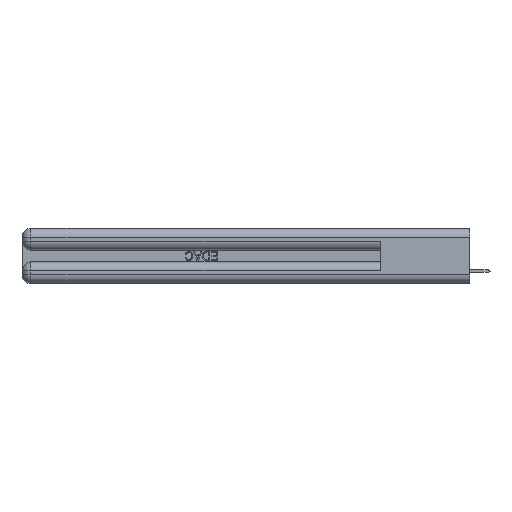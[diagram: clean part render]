
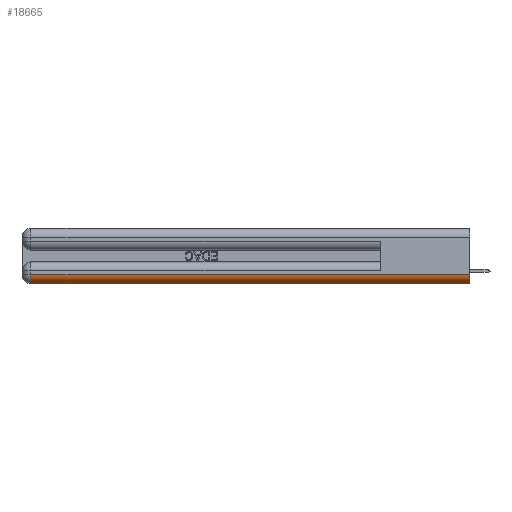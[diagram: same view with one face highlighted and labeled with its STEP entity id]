
A CAD part, left-side view. The second image highlights one B-rep face of the part: STEP entity #18665.
In plain terms, the highlighted cylindrical face has radius 1.524 mm (diameter 3.048 mm), a partial arc.
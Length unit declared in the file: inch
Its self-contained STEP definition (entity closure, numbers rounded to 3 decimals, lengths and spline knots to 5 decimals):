
#1965 = CARTESIAN_POINT ( 'NONE',  ( 0., 0., 0.06 ) ) ;
#2152 = EDGE_CURVE ( 'NONE', #6535, #21701, #43724, .T. ) ;
#2388 = VECTOR ( 'NONE', #12611, 39.37008 ) ;
#3477 = EDGE_CURVE ( 'NONE', #45371, #6535, #14698, .T. ) ;
#5679 = CIRCLE ( 'NONE', #19999, 0.06 ) ;
#5934 = AXIS2_PLACEMENT_3D ( 'NONE', #12713, #40069, #12465 ) ;
#6040 = EDGE_LOOP ( 'NONE', ( #25689, #29995, #38421, #34899 ) ) ;
#6535 = VERTEX_POINT ( 'NONE', #38299 ) ;
#9600 = CARTESIAN_POINT ( 'NONE',  ( 0.06, 3., 0. ) ) ;
#10678 = EDGE_CURVE ( 'NONE', #25312, #45371, #25105, .T. ) ;
#12465 = DIRECTION ( 'NONE',  ( 0., 0., 1. ) ) ;
#12474 = FACE_OUTER_BOUND ( 'NONE', #6040, .T. ) ;
#12611 = DIRECTION ( 'NONE',  ( 0., 1., 0. ) ) ;
#12713 = CARTESIAN_POINT ( 'NONE',  ( 0.06, 0., 0.06 ) ) ;
#14698 = CIRCLE ( 'NONE', #5934, 0.06 ) ;
#17565 = VECTOR ( 'NONE', #29340, 39.37008 ) ;
#18665 = ADVANCED_FACE ( 'NONE', ( #12474 ), #20152, .T. ) ;
#19999 = AXIS2_PLACEMENT_3D ( 'NONE', #34906, #23681, #20188 ) ;
#20152 = CYLINDRICAL_SURFACE ( 'NONE', #43026, 0.06 ) ;
#20188 = DIRECTION ( 'NONE',  ( 0., 0., 1. ) ) ;
#21701 = VERTEX_POINT ( 'NONE', #23457 ) ;
#22611 = CARTESIAN_POINT ( 'NONE',  ( 0., 2.94, 0.06 ) ) ;
#23457 = CARTESIAN_POINT ( 'NONE',  ( 0.06, 2.94, 0. ) ) ;
#23681 = DIRECTION ( 'NONE',  ( 0., 1., 0. ) ) ;
#25105 = LINE ( 'NONE', #47804, #17565 ) ;
#25312 = VERTEX_POINT ( 'NONE', #22611 ) ;
#25689 = ORIENTED_EDGE ( 'NONE', *, *, #3477, .F. ) ;
#27058 = EDGE_CURVE ( 'NONE', #21701, #25312, #5679, .T. ) ;
#27381 = DIRECTION ( 'NONE',  ( 0., 0., 1. ) ) ;
#29340 = DIRECTION ( 'NONE',  ( 0., -1., 0. ) ) ;
#29995 = ORIENTED_EDGE ( 'NONE', *, *, #10678, .F. ) ;
#31393 = CARTESIAN_POINT ( 'NONE',  ( 0.06, 0., 0.06 ) ) ;
#34899 = ORIENTED_EDGE ( 'NONE', *, *, #2152, .F. ) ;
#34906 = CARTESIAN_POINT ( 'NONE',  ( 0.06, 2.94, 0.06 ) ) ;
#38299 = CARTESIAN_POINT ( 'NONE',  ( 0.06, 0., 0. ) ) ;
#38421 = ORIENTED_EDGE ( 'NONE', *, *, #27058, .F. ) ;
#39345 = DIRECTION ( 'NONE',  ( 0., 1., 0. ) ) ;
#40069 = DIRECTION ( 'NONE',  ( 0., -1., 0. ) ) ;
#43026 = AXIS2_PLACEMENT_3D ( 'NONE', #31393, #39345, #27381 ) ;
#43724 = LINE ( 'NONE', #9600, #2388 ) ;
#45371 = VERTEX_POINT ( 'NONE', #1965 ) ;
#47804 = CARTESIAN_POINT ( 'NONE',  ( 0., 0., 0.06 ) ) ;
